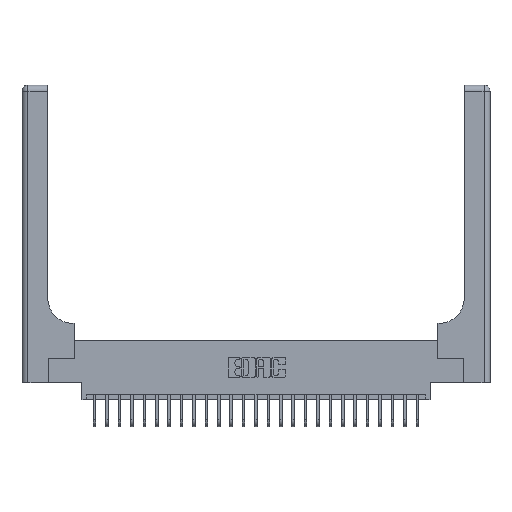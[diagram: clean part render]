
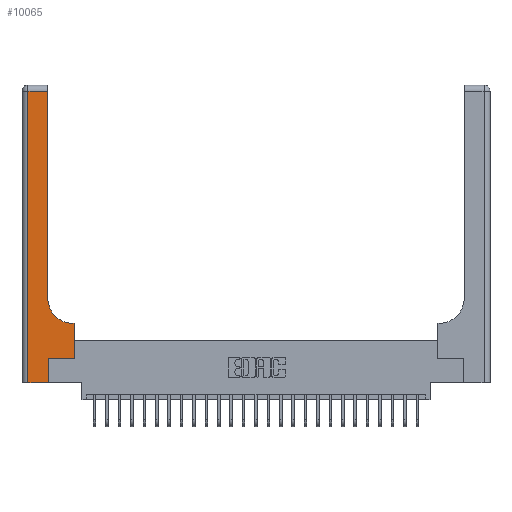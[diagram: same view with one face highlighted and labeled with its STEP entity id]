
A CAD part, top view. The second image highlights one B-rep face of the part: STEP entity #10065.
In plain terms, the highlighted planar face has unit normal (0, 0, 1).
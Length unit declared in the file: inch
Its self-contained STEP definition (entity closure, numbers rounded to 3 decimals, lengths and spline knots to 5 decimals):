
#118 = LINE ( 'NONE', #3639, #22115 ) ;
#796 = DIRECTION ( 'NONE',  ( -1., 0., 0. ) ) ;
#838 = EDGE_LOOP ( 'NONE', ( #15307, #17435, #16423, #12229, #11151, #17935, #12790, #16009, #6172 ) ) ;
#882 = PLANE ( 'NONE',  #24810 ) ;
#945 = VERTEX_POINT ( 'NONE', #15470 ) ;
#1621 = LINE ( 'NONE', #9663, #22929 ) ;
#2070 = VECTOR ( 'NONE', #15267, 39.37008 ) ;
#2182 = CARTESIAN_POINT ( 'NONE',  ( 0.265, 0.25, 0.37 ) ) ;
#2713 = CARTESIAN_POINT ( 'NONE',  ( 0., 3., 0.37 ) ) ;
#3280 = DIRECTION ( 'NONE',  ( 1., 0., 0. ) ) ;
#3375 = DIRECTION ( 'NONE',  ( 0., -1., 0. ) ) ;
#3489 = FACE_OUTER_BOUND ( 'NONE', #838, .T. ) ;
#3639 = CARTESIAN_POINT ( 'NONE',  ( 0.26, 0.6, 0.37 ) ) ;
#6104 = VERTEX_POINT ( 'NONE', #19398 ) ;
#6172 = ORIENTED_EDGE ( 'NONE', *, *, #24774, .T. ) ;
#7105 = DIRECTION ( 'NONE',  ( 1., 0., 0. ) ) ;
#7386 = CARTESIAN_POINT ( 'NONE',  ( 0.265, 0., 0.37 ) ) ;
#8706 = CARTESIAN_POINT ( 'NONE',  ( 0.265, 0., 0.37 ) ) ;
#8969 = DIRECTION ( 'NONE',  ( 0., 1., 0. ) ) ;
#9663 = CARTESIAN_POINT ( 'NONE',  ( 0., 0., 0.37 ) ) ;
#9971 = VERTEX_POINT ( 'NONE', #15006 ) ;
#9976 = EDGE_CURVE ( 'NONE', #19431, #945, #25782, .T. ) ;
#10065 = ADVANCED_FACE ( 'NONE', ( #3489 ), #882, .F. ) ;
#10736 = DIRECTION ( 'NONE',  ( 0., 1., 0. ) ) ;
#10863 = CARTESIAN_POINT ( 'NONE',  ( 0., 2.94, 0.37 ) ) ;
#11151 = ORIENTED_EDGE ( 'NONE', *, *, #25612, .T. ) ;
#11459 = EDGE_CURVE ( 'NONE', #6104, #9971, #11539, .T. ) ;
#11539 = LINE ( 'NONE', #17308, #17348 ) ;
#11663 = VERTEX_POINT ( 'NONE', #16467 ) ;
#11753 = DIRECTION ( 'NONE',  ( -1., 0., 0. ) ) ;
#11941 = VECTOR ( 'NONE', #796, 39.37008 ) ;
#12229 = ORIENTED_EDGE ( 'NONE', *, *, #21966, .T. ) ;
#12538 = LINE ( 'NONE', #13536, #21556 ) ;
#12790 = ORIENTED_EDGE ( 'NONE', *, *, #11459, .T. ) ;
#13536 = CARTESIAN_POINT ( 'NONE',  ( 0.265, 0.25, 0.37 ) ) ;
#13693 = CARTESIAN_POINT ( 'NONE',  ( 0.51, 0.6, 0.37 ) ) ;
#13694 = CARTESIAN_POINT ( 'NONE',  ( 0.51, 0.85, 0.37 ) ) ;
#15006 = CARTESIAN_POINT ( 'NONE',  ( 0.528, 0.6, 0.37 ) ) ;
#15267 = DIRECTION ( 'NONE',  ( 0., 1., 0. ) ) ;
#15307 = ORIENTED_EDGE ( 'NONE', *, *, #19460, .T. ) ;
#15470 = CARTESIAN_POINT ( 'NONE',  ( 0.06, 2.94, 0.37 ) ) ;
#16009 = ORIENTED_EDGE ( 'NONE', *, *, #25040, .T. ) ;
#16189 = DIRECTION ( 'NONE',  ( -1., 0., 0. ) ) ;
#16423 = ORIENTED_EDGE ( 'NONE', *, *, #18757, .T. ) ;
#16467 = CARTESIAN_POINT ( 'NONE',  ( 0.06, 0., 0.37 ) ) ;
#16955 = LINE ( 'NONE', #7386, #2070 ) ;
#17308 = CARTESIAN_POINT ( 'NONE',  ( 0.528, 0.25, 0.37 ) ) ;
#17348 = VECTOR ( 'NONE', #10736, 39.37008 ) ;
#17435 = ORIENTED_EDGE ( 'NONE', *, *, #9976, .T. ) ;
#17724 = VERTEX_POINT ( 'NONE', #8706 ) ;
#17935 = ORIENTED_EDGE ( 'NONE', *, *, #20783, .T. ) ;
#17944 = CIRCLE ( 'NONE', #23256, 0.25 ) ;
#18001 = VECTOR ( 'NONE', #8969, 39.37008 ) ;
#18757 = EDGE_CURVE ( 'NONE', #945, #11663, #22552, .T. ) ;
#19398 = CARTESIAN_POINT ( 'NONE',  ( 0.528, 0.25, 0.37 ) ) ;
#19431 = VERTEX_POINT ( 'NONE', #23486 ) ;
#19460 = EDGE_CURVE ( 'NONE', #19486, #19431, #25086, .T. ) ;
#19486 = VERTEX_POINT ( 'NONE', #21533 ) ;
#19550 = CARTESIAN_POINT ( 'NONE',  ( 0.26, 3., 0.37 ) ) ;
#20625 = VECTOR ( 'NONE', #3375, 39.37008 ) ;
#20783 = EDGE_CURVE ( 'NONE', #23277, #6104, #12538, .T. ) ;
#21453 = CARTESIAN_POINT ( 'NONE',  ( 0.06, 3., 0.37 ) ) ;
#21533 = CARTESIAN_POINT ( 'NONE',  ( 0.26, 0.85, 0.37 ) ) ;
#21556 = VECTOR ( 'NONE', #7105, 39.37008 ) ;
#21672 = DIRECTION ( 'NONE',  ( 1., 0., 0. ) ) ;
#21966 = EDGE_CURVE ( 'NONE', #11663, #17724, #1621, .T. ) ;
#22051 = DIRECTION ( 'NONE',  ( 0., 0., -1. ) ) ;
#22115 = VECTOR ( 'NONE', #16189, 39.37008 ) ;
#22552 = LINE ( 'NONE', #21453, #20625 ) ;
#22929 = VECTOR ( 'NONE', #21672, 39.37008 ) ;
#23256 = AXIS2_PLACEMENT_3D ( 'NONE', #13694, #22051, #3280 ) ;
#23277 = VERTEX_POINT ( 'NONE', #2182 ) ;
#23486 = CARTESIAN_POINT ( 'NONE',  ( 0.26, 2.94, 0.37 ) ) ;
#24774 = EDGE_CURVE ( 'NONE', #26315, #19486, #17944, .T. ) ;
#24810 = AXIS2_PLACEMENT_3D ( 'NONE', #2713, #25435, #11753 ) ;
#25040 = EDGE_CURVE ( 'NONE', #9971, #26315, #118, .T. ) ;
#25086 = LINE ( 'NONE', #19550, #18001 ) ;
#25435 = DIRECTION ( 'NONE',  ( 0., 0., -1. ) ) ;
#25612 = EDGE_CURVE ( 'NONE', #17724, #23277, #16955, .T. ) ;
#25782 = LINE ( 'NONE', #10863, #11941 ) ;
#26315 = VERTEX_POINT ( 'NONE', #13693 ) ;
